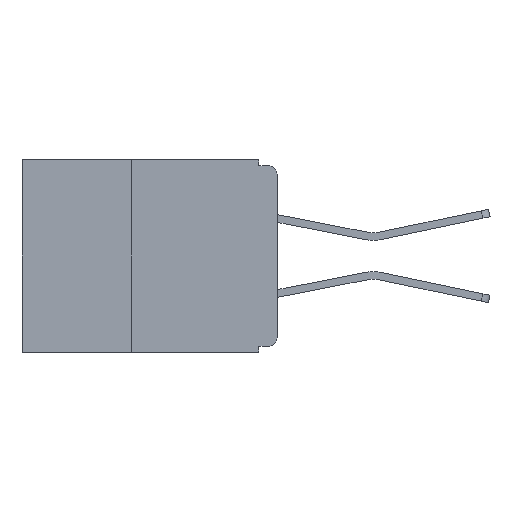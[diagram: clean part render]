
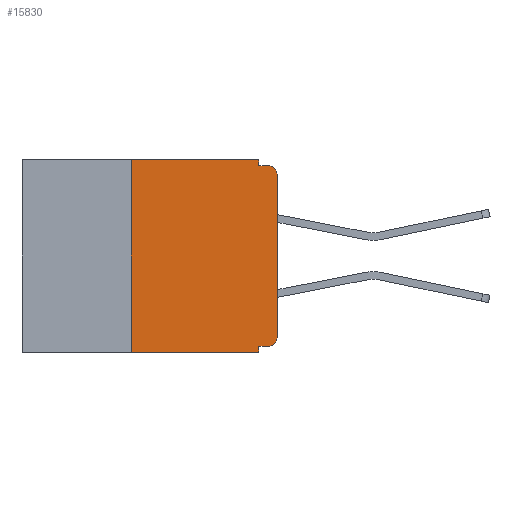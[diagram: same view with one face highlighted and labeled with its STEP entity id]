
A CAD part, left-side view. The second image highlights one B-rep face of the part: STEP entity #15830.
In plain terms, the highlighted planar face has unit normal (-1, 0, 0).
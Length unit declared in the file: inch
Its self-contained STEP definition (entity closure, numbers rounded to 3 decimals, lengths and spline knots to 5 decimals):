
#18 = CARTESIAN_POINT ( 'NONE',  ( 0., 0.015, -0.305 ) ) ;
#340 = EDGE_CURVE ( 'NONE', #23955, #23649, #18343, .T. ) ;
#393 = CARTESIAN_POINT ( 'NONE',  ( 0., 0., -0.305 ) ) ;
#847 = VECTOR ( 'NONE', #4343, 39.37008 ) ;
#1817 = CIRCLE ( 'NONE', #2162, 0.015 ) ;
#1845 = EDGE_LOOP ( 'NONE', ( #18817, #18738, #2550, #3862, #10645, #14719, #6738, #9631, #4141, #9964 ) ) ;
#2162 = AXIS2_PLACEMENT_3D ( 'NONE', #10410, #25096, #12544 ) ;
#2187 = DIRECTION ( 'NONE',  ( 0., 0., -1. ) ) ;
#2283 = EDGE_CURVE ( 'NONE', #26699, #20321, #24686, .T. ) ;
#2533 = VECTOR ( 'NONE', #12607, 39.37008 ) ;
#2550 = ORIENTED_EDGE ( 'NONE', *, *, #340, .F. ) ;
#2774 = DIRECTION ( 'NONE',  ( 0., -1., 0. ) ) ;
#3070 = LINE ( 'NONE', #4711, #19406 ) ;
#3398 = EDGE_CURVE ( 'NONE', #9251, #5147, #3070, .T. ) ;
#3663 = DIRECTION ( 'NONE',  ( 0., 0., -1. ) ) ;
#3862 = ORIENTED_EDGE ( 'NONE', *, *, #17747, .F. ) ;
#3932 = VERTEX_POINT ( 'NONE', #22037 ) ;
#4141 = ORIENTED_EDGE ( 'NONE', *, *, #2283, .F. ) ;
#4281 = VECTOR ( 'NONE', #2774, 39.37008 ) ;
#4343 = DIRECTION ( 'NONE',  ( 0., -1., 0. ) ) ;
#4654 = DIRECTION ( 'NONE',  ( 0., 0., 1. ) ) ;
#4711 = CARTESIAN_POINT ( 'NONE',  ( 0., 0., 0. ) ) ;
#4725 = DIRECTION ( 'NONE',  ( 0., -1., 0. ) ) ;
#5147 = VERTEX_POINT ( 'NONE', #7167 ) ;
#5440 = CARTESIAN_POINT ( 'NONE',  ( 0., 0.25, -0.33 ) ) ;
#6738 = ORIENTED_EDGE ( 'NONE', *, *, #8687, .T. ) ;
#7167 = CARTESIAN_POINT ( 'NONE',  ( 0., 0., -0.025 ) ) ;
#7755 = CARTESIAN_POINT ( 'NONE',  ( 0., 0.031, -0.33 ) ) ;
#7894 = CARTESIAN_POINT ( 'NONE',  ( 0., 0.031, -0.33 ) ) ;
#8051 = LINE ( 'NONE', #19606, #19345 ) ;
#8244 = LINE ( 'NONE', #25147, #2533 ) ;
#8494 = DIRECTION ( 'NONE',  ( 0., 1., 0. ) ) ;
#8687 = EDGE_CURVE ( 'NONE', #26236, #12989, #24814, .T. ) ;
#8701 = CARTESIAN_POINT ( 'NONE',  ( 0., 0., -0.32 ) ) ;
#9251 = VERTEX_POINT ( 'NONE', #393 ) ;
#9631 = ORIENTED_EDGE ( 'NONE', *, *, #15800, .F. ) ;
#9964 = ORIENTED_EDGE ( 'NONE', *, *, #13254, .T. ) ;
#10410 = CARTESIAN_POINT ( 'NONE',  ( 0., 0.015, -0.025 ) ) ;
#10645 = ORIENTED_EDGE ( 'NONE', *, *, #27154, .F. ) ;
#11366 = CARTESIAN_POINT ( 'NONE',  ( 0., 0.25, 0. ) ) ;
#12089 = LINE ( 'NONE', #19447, #27393 ) ;
#12544 = DIRECTION ( 'NONE',  ( 0., 0., -1. ) ) ;
#12607 = DIRECTION ( 'NONE',  ( 0., 0., -1. ) ) ;
#12989 = VERTEX_POINT ( 'NONE', #7755 ) ;
#13254 = EDGE_CURVE ( 'NONE', #26699, #9251, #23076, .T. ) ;
#14719 = ORIENTED_EDGE ( 'NONE', *, *, #24749, .F. ) ;
#15000 = DIRECTION ( 'NONE',  ( -1., 0., 0. ) ) ;
#15234 = CARTESIAN_POINT ( 'NONE',  ( 0., 0.031, -0.01 ) ) ;
#15800 = EDGE_CURVE ( 'NONE', #20321, #12989, #18011, .T. ) ;
#15830 = ADVANCED_FACE ( 'NONE', ( #22925 ), #24788, .F. ) ;
#16273 = CARTESIAN_POINT ( 'NONE',  ( 0., 0.015, -0.01 ) ) ;
#16451 = DIRECTION ( 'NONE',  ( 1., 0., 0. ) ) ;
#16759 = VERTEX_POINT ( 'NONE', #11366 ) ;
#17470 = AXIS2_PLACEMENT_3D ( 'NONE', #26830, #16451, #3663 ) ;
#17747 = EDGE_CURVE ( 'NONE', #3932, #23955, #8244, .T. ) ;
#18011 = LINE ( 'NONE', #7894, #18666 ) ;
#18343 = LINE ( 'NONE', #26339, #847 ) ;
#18666 = VECTOR ( 'NONE', #22705, 39.37008 ) ;
#18738 = ORIENTED_EDGE ( 'NONE', *, *, #20823, .T. ) ;
#18817 = ORIENTED_EDGE ( 'NONE', *, *, #3398, .T. ) ;
#19150 = VECTOR ( 'NONE', #8494, 39.37008 ) ;
#19345 = VECTOR ( 'NONE', #4725, 39.37008 ) ;
#19406 = VECTOR ( 'NONE', #4654, 39.37008 ) ;
#19447 = CARTESIAN_POINT ( 'NONE',  ( 0., 0.25, -0.33 ) ) ;
#19606 = CARTESIAN_POINT ( 'NONE',  ( 0., 0.437, 0. ) ) ;
#20321 = VERTEX_POINT ( 'NONE', #25475 ) ;
#20823 = EDGE_CURVE ( 'NONE', #5147, #23649, #1817, .T. ) ;
#21539 = DIRECTION ( 'NONE',  ( 0., 0., 1. ) ) ;
#22037 = CARTESIAN_POINT ( 'NONE',  ( 0., 0.031, 0. ) ) ;
#22705 = DIRECTION ( 'NONE',  ( 0., 0., -1. ) ) ;
#22925 = FACE_OUTER_BOUND ( 'NONE', #1845, .T. ) ;
#23076 = CIRCLE ( 'NONE', #26321, 0.015 ) ;
#23649 = VERTEX_POINT ( 'NONE', #16273 ) ;
#23955 = VERTEX_POINT ( 'NONE', #15234 ) ;
#24200 = CARTESIAN_POINT ( 'NONE',  ( 0., 0.015, -0.32 ) ) ;
#24686 = LINE ( 'NONE', #8701, #19150 ) ;
#24749 = EDGE_CURVE ( 'NONE', #26236, #16759, #12089, .T. ) ;
#24788 = PLANE ( 'NONE',  #17470 ) ;
#24814 = LINE ( 'NONE', #26069, #4281 ) ;
#25096 = DIRECTION ( 'NONE',  ( -1., 0., 0. ) ) ;
#25147 = CARTESIAN_POINT ( 'NONE',  ( 0., 0.031, 0. ) ) ;
#25475 = CARTESIAN_POINT ( 'NONE',  ( 0., 0.031, -0.32 ) ) ;
#26069 = CARTESIAN_POINT ( 'NONE',  ( 0., 0.437, -0.33 ) ) ;
#26236 = VERTEX_POINT ( 'NONE', #5440 ) ;
#26321 = AXIS2_PLACEMENT_3D ( 'NONE', #18, #15000, #2187 ) ;
#26339 = CARTESIAN_POINT ( 'NONE',  ( 0., 0., -0.01 ) ) ;
#26699 = VERTEX_POINT ( 'NONE', #24200 ) ;
#26830 = CARTESIAN_POINT ( 'NONE',  ( 0., 0.437, 0. ) ) ;
#27154 = EDGE_CURVE ( 'NONE', #16759, #3932, #8051, .T. ) ;
#27393 = VECTOR ( 'NONE', #21539, 39.37008 ) ;
